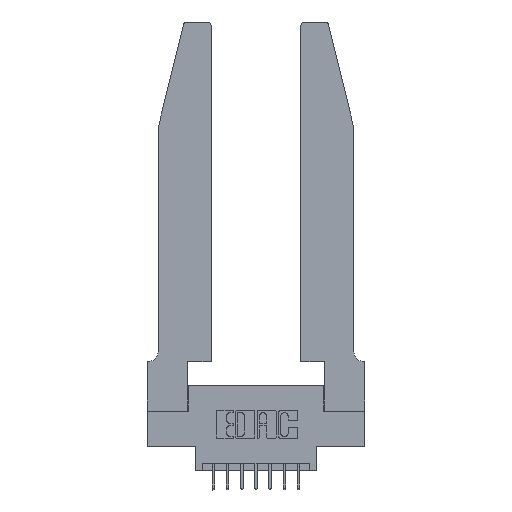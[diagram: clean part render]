
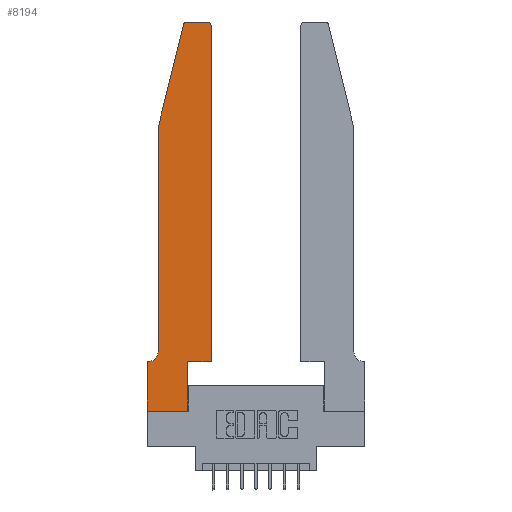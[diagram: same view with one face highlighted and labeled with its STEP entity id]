
A CAD part, top view. The second image highlights one B-rep face of the part: STEP entity #8194.
In plain terms, the highlighted planar face has unit normal (0, 0, 1).
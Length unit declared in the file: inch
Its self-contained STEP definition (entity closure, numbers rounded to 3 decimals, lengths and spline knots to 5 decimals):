
#337 = ORIENTED_EDGE ( 'NONE', *, *, #2399, .T. ) ;
#540 = EDGE_CURVE ( 'NONE', #7472, #9647, #15071, .T. ) ;
#600 = CIRCLE ( 'NONE', #2563, 0.03 ) ;
#667 = LINE ( 'NONE', #4307, #14456 ) ;
#707 = AXIS2_PLACEMENT_3D ( 'NONE', #5706, #10646, #11439 ) ;
#857 = VECTOR ( 'NONE', #3446, 39.37008 ) ;
#1048 = EDGE_CURVE ( 'NONE', #14784, #7472, #15132, .T. ) ;
#1161 = ORIENTED_EDGE ( 'NONE', *, *, #8570, .T. ) ;
#1249 = ORIENTED_EDGE ( 'NONE', *, *, #4077, .T. ) ;
#1338 = EDGE_CURVE ( 'NONE', #2824, #11196, #600, .T. ) ;
#1780 = VECTOR ( 'NONE', #9002, 39.37008 ) ;
#2024 = DIRECTION ( 'NONE',  ( 0., -1., 0. ) ) ;
#2135 = CARTESIAN_POINT ( 'NONE',  ( 0.284, 2.75, 0.37 ) ) ;
#2158 = CIRCLE ( 'NONE', #8047, 0.07 ) ;
#2272 = ORIENTED_EDGE ( 'NONE', *, *, #10179, .T. ) ;
#2366 = EDGE_LOOP ( 'NONE', ( #4244, #12294, #4597, #337, #1161, #5517, #14214, #2272, #6143, #8263, #1249, #7889 ) ) ;
#2399 = EDGE_CURVE ( 'NONE', #13476, #7509, #3185, .T. ) ;
#2459 = DIRECTION ( 'NONE',  ( 1., 0., 0. ) ) ;
#2484 = DIRECTION ( 'NONE',  ( 0., 0., 1. ) ) ;
#2563 = AXIS2_PLACEMENT_3D ( 'NONE', #7814, #14886, #14961 ) ;
#2780 = EDGE_CURVE ( 'NONE', #11196, #13476, #667, .T. ) ;
#2824 = VERTEX_POINT ( 'NONE', #2135 ) ;
#3185 = LINE ( 'NONE', #11449, #11279 ) ;
#3446 = DIRECTION ( 'NONE',  ( 1., 0., 0. ) ) ;
#3588 = CIRCLE ( 'NONE', #5061, 0.03 ) ;
#3679 = VECTOR ( 'NONE', #2459, 39.37008 ) ;
#3713 = EDGE_CURVE ( 'NONE', #8947, #10495, #7966, .T. ) ;
#3803 = CARTESIAN_POINT ( 'NONE',  ( 0.4505, 2.72, 0.37 ) ) ;
#3848 = VECTOR ( 'NONE', #7925, 39.37008 ) ;
#3862 = LINE ( 'NONE', #7439, #3679 ) ;
#3874 = CARTESIAN_POINT ( 'NONE',  ( 0., 0., 0.37 ) ) ;
#4077 = EDGE_CURVE ( 'NONE', #10495, #11082, #4185, .T. ) ;
#4099 = CARTESIAN_POINT ( 'NONE',  ( 0.25487, 2.72718, 0.37 ) ) ;
#4185 = LINE ( 'NONE', #12383, #3848 ) ;
#4229 = EDGE_CURVE ( 'NONE', #11082, #13289, #3588, .T. ) ;
#4244 = ORIENTED_EDGE ( 'NONE', *, *, #4557, .T. ) ;
#4307 = CARTESIAN_POINT ( 'NONE',  ( 0.0755, 2., 0.37 ) ) ;
#4557 = EDGE_CURVE ( 'NONE', #13289, #2824, #12403, .T. ) ;
#4575 = VERTEX_POINT ( 'NONE', #5425 ) ;
#4597 = ORIENTED_EDGE ( 'NONE', *, *, #2780, .T. ) ;
#4598 = CARTESIAN_POINT ( 'NONE',  ( 0.4505, 0.35, 0.37 ) ) ;
#4615 = CARTESIAN_POINT ( 'NONE',  ( 0.0755, 0.35, 0.37 ) ) ;
#4861 = DIRECTION ( 'NONE',  ( 0., 0., -1. ) ) ;
#5061 = AXIS2_PLACEMENT_3D ( 'NONE', #13162, #2484, #7167 ) ;
#5086 = DIRECTION ( 'NONE',  ( -1., 0., 0. ) ) ;
#5425 = CARTESIAN_POINT ( 'NONE',  ( 0.2865, 0., 0.37 ) ) ;
#5512 = VECTOR ( 'NONE', #12461, 39.37008 ) ;
#5517 = ORIENTED_EDGE ( 'NONE', *, *, #1048, .T. ) ;
#5706 = CARTESIAN_POINT ( 'NONE',  ( 0., 0.35, 0.37 ) ) ;
#6143 = ORIENTED_EDGE ( 'NONE', *, *, #13514, .T. ) ;
#6486 = CARTESIAN_POINT ( 'NONE',  ( 0.0055, 0.35, 0.37 ) ) ;
#7167 = DIRECTION ( 'NONE',  ( 1., 0., 0. ) ) ;
#7233 = CARTESIAN_POINT ( 'NONE',  ( 0.4505, 0.35, 0.37 ) ) ;
#7439 = CARTESIAN_POINT ( 'NONE',  ( 0., 0., 0.37 ) ) ;
#7472 = VERTEX_POINT ( 'NONE', #10631 ) ;
#7509 = VERTEX_POINT ( 'NONE', #8400 ) ;
#7564 = CARTESIAN_POINT ( 'NONE',  ( 0.2865, 0.35, 0.37 ) ) ;
#7620 = LINE ( 'NONE', #11229, #1780 ) ;
#7730 = VECTOR ( 'NONE', #9283, 39.37008 ) ;
#7814 = CARTESIAN_POINT ( 'NONE',  ( 0.284, 2.72, 0.37 ) ) ;
#7889 = ORIENTED_EDGE ( 'NONE', *, *, #4229, .T. ) ;
#7923 = PLANE ( 'NONE',  #707 ) ;
#7925 = DIRECTION ( 'NONE',  ( 0., 1., 0. ) ) ;
#7966 = LINE ( 'NONE', #4598, #857 ) ;
#8047 = AXIS2_PLACEMENT_3D ( 'NONE', #9765, #4861, #5086 ) ;
#8194 = ADVANCED_FACE ( 'NONE', ( #11043 ), #7923, .T. ) ;
#8263 = ORIENTED_EDGE ( 'NONE', *, *, #3713, .T. ) ;
#8400 = CARTESIAN_POINT ( 'NONE',  ( 0.0755, 0.42, 0.37 ) ) ;
#8570 = EDGE_CURVE ( 'NONE', #7509, #14784, #2158, .T. ) ;
#8947 = VERTEX_POINT ( 'NONE', #7564 ) ;
#9002 = DIRECTION ( 'NONE',  ( 0., 1., 0. ) ) ;
#9086 = DIRECTION ( 'NONE',  ( -1., 0., 0. ) ) ;
#9283 = DIRECTION ( 'NONE',  ( -1., 0., 0. ) ) ;
#9630 = CARTESIAN_POINT ( 'NONE',  ( 0.0755, 2., 0.37 ) ) ;
#9647 = VERTEX_POINT ( 'NONE', #3874 ) ;
#9765 = CARTESIAN_POINT ( 'NONE',  ( 0.0055, 0.42, 0.37 ) ) ;
#10179 = EDGE_CURVE ( 'NONE', #9647, #4575, #3862, .T. ) ;
#10468 = CARTESIAN_POINT ( 'NONE',  ( 0.4205, 2.75, 0.37 ) ) ;
#10495 = VERTEX_POINT ( 'NONE', #7233 ) ;
#10631 = CARTESIAN_POINT ( 'NONE',  ( 0., 0.35, 0.37 ) ) ;
#10646 = DIRECTION ( 'NONE',  ( 0., 0., 1. ) ) ;
#11043 = FACE_OUTER_BOUND ( 'NONE', #2366, .T. ) ;
#11082 = VERTEX_POINT ( 'NONE', #3803 ) ;
#11196 = VERTEX_POINT ( 'NONE', #4099 ) ;
#11229 = CARTESIAN_POINT ( 'NONE',  ( 0.2865, 0.35, 0.37 ) ) ;
#11279 = VECTOR ( 'NONE', #2024, 39.37008 ) ;
#11418 = DIRECTION ( 'NONE',  ( -0.239, -0.971, 0. ) ) ;
#11439 = DIRECTION ( 'NONE',  ( 1., 0., 0. ) ) ;
#11449 = CARTESIAN_POINT ( 'NONE',  ( 0.0755, 2., 0.37 ) ) ;
#12294 = ORIENTED_EDGE ( 'NONE', *, *, #1338, .T. ) ;
#12383 = CARTESIAN_POINT ( 'NONE',  ( 0.4505, 0.35, 0.37 ) ) ;
#12403 = LINE ( 'NONE', #14935, #14872 ) ;
#12461 = DIRECTION ( 'NONE',  ( 0., -1., 0. ) ) ;
#13162 = CARTESIAN_POINT ( 'NONE',  ( 0.4205, 2.72, 0.37 ) ) ;
#13289 = VERTEX_POINT ( 'NONE', #10468 ) ;
#13476 = VERTEX_POINT ( 'NONE', #9630 ) ;
#13514 = EDGE_CURVE ( 'NONE', #4575, #8947, #7620, .T. ) ;
#14214 = ORIENTED_EDGE ( 'NONE', *, *, #540, .T. ) ;
#14456 = VECTOR ( 'NONE', #11418, 39.37008 ) ;
#14784 = VERTEX_POINT ( 'NONE', #6486 ) ;
#14848 = CARTESIAN_POINT ( 'NONE',  ( 0., 0., 0.37 ) ) ;
#14872 = VECTOR ( 'NONE', #9086, 39.37008 ) ;
#14886 = DIRECTION ( 'NONE',  ( 0., 0., 1. ) ) ;
#14935 = CARTESIAN_POINT ( 'NONE',  ( 0.2605, 2.75, 0.37 ) ) ;
#14961 = DIRECTION ( 'NONE',  ( 1., 0., 0. ) ) ;
#15071 = LINE ( 'NONE', #14848, #5512 ) ;
#15132 = LINE ( 'NONE', #4615, #7730 ) ;
